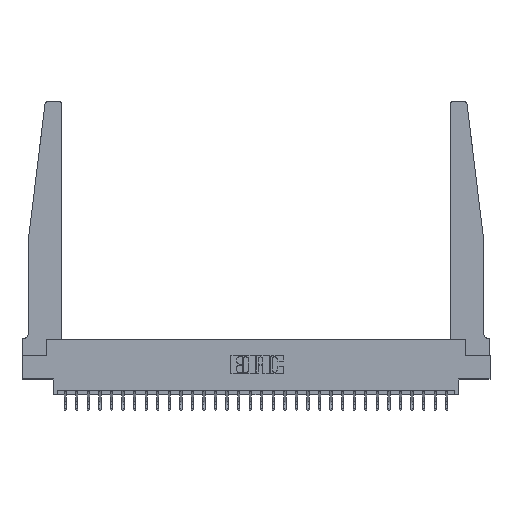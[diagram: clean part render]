
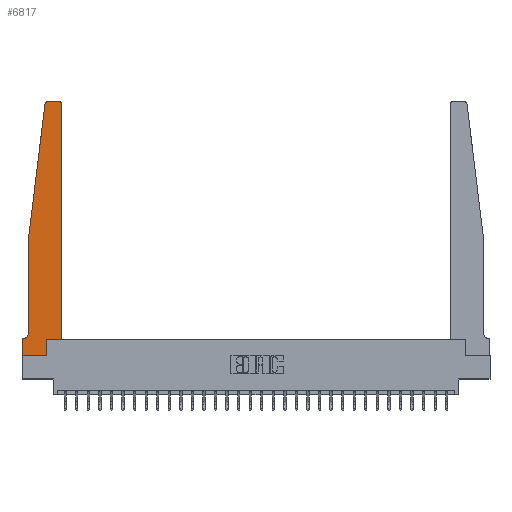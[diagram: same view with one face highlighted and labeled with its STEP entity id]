
A CAD part, top view. The second image highlights one B-rep face of the part: STEP entity #6817.
In plain terms, the highlighted planar face has unit normal (0, 0, 1).
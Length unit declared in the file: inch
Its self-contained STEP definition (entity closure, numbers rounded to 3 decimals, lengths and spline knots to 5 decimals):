
#2 = CARTESIAN_POINT ( 'NONE',  ( 0.24675, 2.72367, 0.37 ) ) ;
#67 = EDGE_CURVE ( 'NONE', #2839, #1694, #6463, .T. ) ;
#218 = VERTEX_POINT ( 'NONE', #547 ) ;
#547 = CARTESIAN_POINT ( 'NONE',  ( 0.425, 0.18, 0.37 ) ) ;
#814 = ORIENTED_EDGE ( 'NONE', *, *, #28179, .T. ) ;
#944 = VECTOR ( 'NONE', #25507, 39.37008 ) ;
#1487 = CIRCLE ( 'NONE', #1876, 0.05 ) ;
#1530 = VERTEX_POINT ( 'NONE', #7929 ) ;
#1689 = EDGE_CURVE ( 'NONE', #18223, #16966, #16600, .T. ) ;
#1694 = VERTEX_POINT ( 'NONE', #21625 ) ;
#1810 = CARTESIAN_POINT ( 'NONE',  ( 0.065, 1.25, 0.37 ) ) ;
#1876 = AXIS2_PLACEMENT_3D ( 'NONE', #25884, #12790, #28074 ) ;
#2066 = EDGE_CURVE ( 'NONE', #16966, #7706, #15526, .T. ) ;
#2490 = CARTESIAN_POINT ( 'NONE',  ( 0.395, 2.72, 0.37 ) ) ;
#2839 = VERTEX_POINT ( 'NONE', #9822 ) ;
#2893 = DIRECTION ( 'NONE',  ( 0., -1., 0. ) ) ;
#3153 = VECTOR ( 'NONE', #11429, 39.37008 ) ;
#3392 = PLANE ( 'NONE',  #21899 ) ;
#3629 = DIRECTION ( 'NONE',  ( -1., 0., 0. ) ) ;
#3756 = DIRECTION ( 'NONE',  ( 0., 0., 1. ) ) ;
#3894 = EDGE_CURVE ( 'NONE', #14353, #218, #21616, .T. ) ;
#4654 = CARTESIAN_POINT ( 'NONE',  ( 0.015, 0.1875, 0.37 ) ) ;
#4733 = DIRECTION ( 'NONE',  ( 1., 0., 0. ) ) ;
#4760 = VECTOR ( 'NONE', #18372, 39.37008 ) ;
#5389 = EDGE_CURVE ( 'NONE', #11907, #1530, #20153, .T. ) ;
#5511 = CARTESIAN_POINT ( 'NONE',  ( 0., 0.1875, 0.37 ) ) ;
#5532 = LINE ( 'NONE', #21036, #28161 ) ;
#5612 = DIRECTION ( 'NONE',  ( 0., 0., 1. ) ) ;
#6463 = LINE ( 'NONE', #17795, #10964 ) ;
#6817 = ADVANCED_FACE ( 'NONE', ( #20766 ), #3392, .T. ) ;
#7084 = ORIENTED_EDGE ( 'NONE', *, *, #14820, .T. ) ;
#7500 = LINE ( 'NONE', #7968, #944 ) ;
#7706 = VERTEX_POINT ( 'NONE', #17767 ) ;
#7929 = CARTESIAN_POINT ( 'NONE',  ( 0., 0.1875, 0.37 ) ) ;
#7968 = CARTESIAN_POINT ( 'NONE',  ( 0.2605, 0.18, 0.37 ) ) ;
#8080 = ORIENTED_EDGE ( 'NONE', *, *, #2066, .T. ) ;
#8407 = LINE ( 'NONE', #27004, #19384 ) ;
#9212 = CARTESIAN_POINT ( 'NONE',  ( 0.425, 0.18, 0.37 ) ) ;
#9299 = CARTESIAN_POINT ( 'NONE',  ( 0.425, 2.72, 0.37 ) ) ;
#9758 = CARTESIAN_POINT ( 'NONE',  ( 0.065, 0.1875, 0.37 ) ) ;
#9822 = CARTESIAN_POINT ( 'NONE',  ( 0., 0., 0.37 ) ) ;
#10238 = EDGE_CURVE ( 'NONE', #25969, #18223, #11947, .T. ) ;
#10240 = ORIENTED_EDGE ( 'NONE', *, *, #10238, .T. ) ;
#10611 = DIRECTION ( 'NONE',  ( 0., -1., 0. ) ) ;
#10740 = VECTOR ( 'NONE', #23852, 39.37008 ) ;
#10964 = VECTOR ( 'NONE', #19998, 39.37008 ) ;
#11429 = DIRECTION ( 'NONE',  ( 0., 1., 0. ) ) ;
#11536 = ORIENTED_EDGE ( 'NONE', *, *, #17575, .T. ) ;
#11593 = ORIENTED_EDGE ( 'NONE', *, *, #19576, .T. ) ;
#11696 = EDGE_CURVE ( 'NONE', #7706, #11907, #1487, .T. ) ;
#11907 = VERTEX_POINT ( 'NONE', #4654 ) ;
#11947 = CIRCLE ( 'NONE', #16486, 0.03 ) ;
#12019 = CARTESIAN_POINT ( 'NONE',  ( 0.065, 1.25, 0.37 ) ) ;
#12564 = ORIENTED_EDGE ( 'NONE', *, *, #1689, .T. ) ;
#12790 = DIRECTION ( 'NONE',  ( 0., 0., -1. ) ) ;
#13657 = VECTOR ( 'NONE', #27257, 39.37008 ) ;
#13943 = ORIENTED_EDGE ( 'NONE', *, *, #5389, .T. ) ;
#14353 = VERTEX_POINT ( 'NONE', #26954 ) ;
#14820 = EDGE_CURVE ( 'NONE', #218, #20205, #27202, .T. ) ;
#15321 = ORIENTED_EDGE ( 'NONE', *, *, #67, .T. ) ;
#15415 = CIRCLE ( 'NONE', #27557, 0.03 ) ;
#15526 = LINE ( 'NONE', #19315, #25088 ) ;
#16055 = ORIENTED_EDGE ( 'NONE', *, *, #11696, .T. ) ;
#16486 = AXIS2_PLACEMENT_3D ( 'NONE', #16984, #3756, #19150 ) ;
#16600 = LINE ( 'NONE', #1810, #10740 ) ;
#16966 = VERTEX_POINT ( 'NONE', #12019 ) ;
#16984 = CARTESIAN_POINT ( 'NONE',  ( 0.27653, 2.72, 0.37 ) ) ;
#17211 = EDGE_CURVE ( 'NONE', #1694, #14353, #7500, .T. ) ;
#17575 = EDGE_CURVE ( 'NONE', #20205, #23867, #15415, .T. ) ;
#17767 = CARTESIAN_POINT ( 'NONE',  ( 0.065, 0.2375, 0.37 ) ) ;
#17795 = CARTESIAN_POINT ( 'NONE',  ( 0., 0., 0.37 ) ) ;
#17926 = DIRECTION ( 'NONE',  ( 0., 0., 1. ) ) ;
#18223 = VERTEX_POINT ( 'NONE', #2 ) ;
#18372 = DIRECTION ( 'NONE',  ( 1., 0., 0. ) ) ;
#19150 = DIRECTION ( 'NONE',  ( 1., 0., 0. ) ) ;
#19315 = CARTESIAN_POINT ( 'NONE',  ( 0.065, 1.25, 0.37 ) ) ;
#19384 = VECTOR ( 'NONE', #2893, 39.37008 ) ;
#19576 = EDGE_CURVE ( 'NONE', #1530, #2839, #8407, .T. ) ;
#19794 = EDGE_LOOP ( 'NONE', ( #814, #10240, #12564, #8080, #16055, #13943, #11593, #15321, #23259, #28289, #7084, #11536 ) ) ;
#19998 = DIRECTION ( 'NONE',  ( 1., 0., 0. ) ) ;
#20138 = CARTESIAN_POINT ( 'NONE',  ( 0.27653, 2.75, 0.37 ) ) ;
#20153 = LINE ( 'NONE', #9758, #13657 ) ;
#20205 = VERTEX_POINT ( 'NONE', #9299 ) ;
#20766 = FACE_OUTER_BOUND ( 'NONE', #19794, .T. ) ;
#20979 = DIRECTION ( 'NONE',  ( 1., 0., 0. ) ) ;
#21036 = CARTESIAN_POINT ( 'NONE',  ( 0.25, 2.75, 0.37 ) ) ;
#21616 = LINE ( 'NONE', #22772, #4760 ) ;
#21625 = CARTESIAN_POINT ( 'NONE',  ( 0.2605, 0., 0.37 ) ) ;
#21899 = AXIS2_PLACEMENT_3D ( 'NONE', #5511, #5612, #20979 ) ;
#22772 = CARTESIAN_POINT ( 'NONE',  ( 0.425, 0.18, 0.37 ) ) ;
#23259 = ORIENTED_EDGE ( 'NONE', *, *, #17211, .T. ) ;
#23852 = DIRECTION ( 'NONE',  ( -0.122, -0.992, 0. ) ) ;
#23867 = VERTEX_POINT ( 'NONE', #26190 ) ;
#25088 = VECTOR ( 'NONE', #10611, 39.37008 ) ;
#25507 = DIRECTION ( 'NONE',  ( 0., 1., 0. ) ) ;
#25884 = CARTESIAN_POINT ( 'NONE',  ( 0.015, 0.2375, 0.37 ) ) ;
#25969 = VERTEX_POINT ( 'NONE', #20138 ) ;
#26190 = CARTESIAN_POINT ( 'NONE',  ( 0.395, 2.75, 0.37 ) ) ;
#26954 = CARTESIAN_POINT ( 'NONE',  ( 0.2605, 0.18, 0.37 ) ) ;
#27004 = CARTESIAN_POINT ( 'NONE',  ( 0., 0., 0.37 ) ) ;
#27202 = LINE ( 'NONE', #9212, #3153 ) ;
#27257 = DIRECTION ( 'NONE',  ( -1., 0., 0. ) ) ;
#27557 = AXIS2_PLACEMENT_3D ( 'NONE', #2490, #17926, #4733 ) ;
#28074 = DIRECTION ( 'NONE',  ( -1., 0., 0. ) ) ;
#28161 = VECTOR ( 'NONE', #3629, 39.37008 ) ;
#28179 = EDGE_CURVE ( 'NONE', #23867, #25969, #5532, .T. ) ;
#28289 = ORIENTED_EDGE ( 'NONE', *, *, #3894, .T. ) ;
